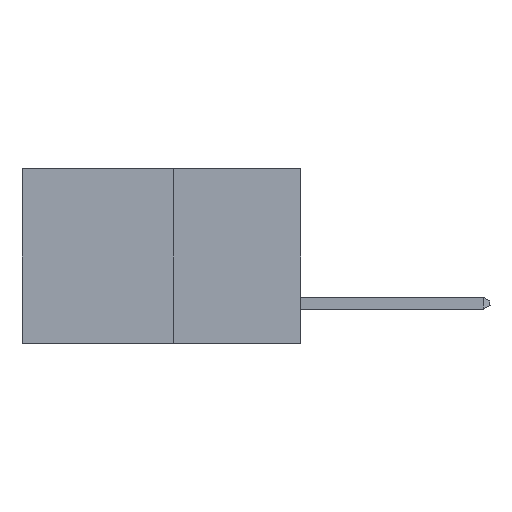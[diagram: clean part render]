
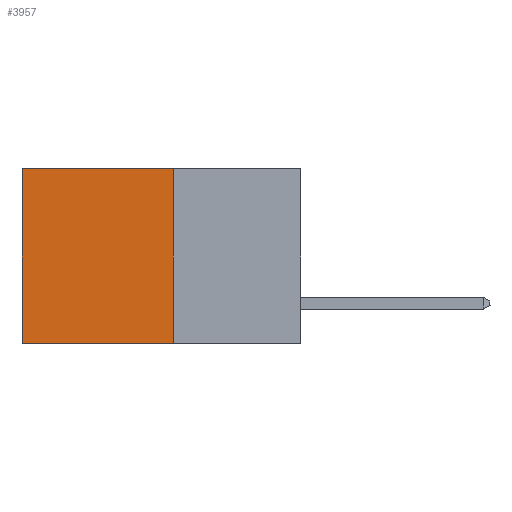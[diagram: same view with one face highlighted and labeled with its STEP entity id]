
A CAD part, left-side view. The second image highlights one B-rep face of the part: STEP entity #3957.
In plain terms, the highlighted planar face has unit normal (-1, 0, 0).
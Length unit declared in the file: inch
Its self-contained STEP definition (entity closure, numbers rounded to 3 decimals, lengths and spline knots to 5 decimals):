
#230 = CARTESIAN_POINT ( 'NONE',  ( 0.277, 0.27, 0. ) ) ;
#341 = CARTESIAN_POINT ( 'NONE',  ( 0.277, 0.59, 0. ) ) ;
#1220 = PLANE ( 'NONE',  #7655 ) ;
#1552 = EDGE_CURVE ( 'NONE', #28810, #23017, #10580, .T. ) ;
#2754 = ORIENTED_EDGE ( 'NONE', *, *, #29210, .T. ) ;
#3629 = DIRECTION ( 'NONE',  ( 1., 0., 0. ) ) ;
#3957 = ADVANCED_FACE ( 'NONE', ( #7433 ), #1220, .F. ) ;
#4206 = CARTESIAN_POINT ( 'NONE',  ( 0.277, 0.27, -0.37 ) ) ;
#6127 = CARTESIAN_POINT ( 'NONE',  ( 0.277, 0.59, -0.37 ) ) ;
#7433 = FACE_OUTER_BOUND ( 'NONE', #20163, .T. ) ;
#7655 = AXIS2_PLACEMENT_3D ( 'NONE', #27316, #3629, #23700 ) ;
#8037 = ORIENTED_EDGE ( 'NONE', *, *, #9283, .T. ) ;
#9215 = ORIENTED_EDGE ( 'NONE', *, *, #23869, .F. ) ;
#9283 = EDGE_CURVE ( 'NONE', #28810, #14329, #25653, .T. ) ;
#10580 = LINE ( 'NONE', #28016, #11988 ) ;
#10627 = CARTESIAN_POINT ( 'NONE',  ( 0.277, 0.27, 0. ) ) ;
#11629 = CARTESIAN_POINT ( 'NONE',  ( 0.277, 0.27, -0.37 ) ) ;
#11988 = VECTOR ( 'NONE', #28047, 39.37008 ) ;
#12817 = VECTOR ( 'NONE', #16220, 39.37008 ) ;
#12828 = VERTEX_POINT ( 'NONE', #6127 ) ;
#12893 = CARTESIAN_POINT ( 'NONE',  ( 0.277, 0.59, -0.37 ) ) ;
#13060 = VECTOR ( 'NONE', #22011, 39.37008 ) ;
#13521 = LINE ( 'NONE', #11629, #12817 ) ;
#14329 = VERTEX_POINT ( 'NONE', #341 ) ;
#14365 = VECTOR ( 'NONE', #26436, 39.37008 ) ;
#16220 = DIRECTION ( 'NONE',  ( 0., 1., 0. ) ) ;
#20163 = EDGE_LOOP ( 'NONE', ( #2754, #9215, #22734, #8037 ) ) ;
#22011 = DIRECTION ( 'NONE',  ( 0., 0., -1. ) ) ;
#22734 = ORIENTED_EDGE ( 'NONE', *, *, #1552, .F. ) ;
#23017 = VERTEX_POINT ( 'NONE', #4206 ) ;
#23700 = DIRECTION ( 'NONE',  ( 0., 0., -1. ) ) ;
#23869 = EDGE_CURVE ( 'NONE', #23017, #12828, #13521, .T. ) ;
#25653 = LINE ( 'NONE', #10627, #14365 ) ;
#25779 = LINE ( 'NONE', #12893, #13060 ) ;
#26436 = DIRECTION ( 'NONE',  ( 0., 1., 0. ) ) ;
#27316 = CARTESIAN_POINT ( 'NONE',  ( 0.277, 0.27, -0.37 ) ) ;
#28016 = CARTESIAN_POINT ( 'NONE',  ( 0.277, 0.27, -0.37 ) ) ;
#28047 = DIRECTION ( 'NONE',  ( 0., 0., -1. ) ) ;
#28810 = VERTEX_POINT ( 'NONE', #230 ) ;
#29210 = EDGE_CURVE ( 'NONE', #14329, #12828, #25779, .T. ) ;
